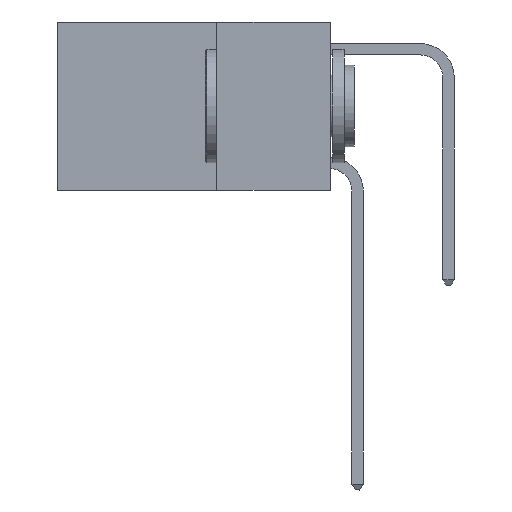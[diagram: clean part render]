
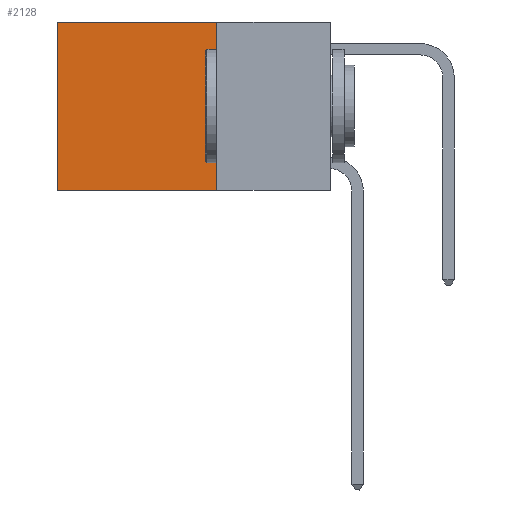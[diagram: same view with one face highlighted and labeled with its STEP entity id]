
A CAD part, left-side view. The second image highlights one B-rep face of the part: STEP entity #2128.
In plain terms, the highlighted planar face has unit normal (-1, 0, 0).
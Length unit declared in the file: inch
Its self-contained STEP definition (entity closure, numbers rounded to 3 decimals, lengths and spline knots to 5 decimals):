
#914 = EDGE_CURVE ( 'NONE', #6549, #8382, #4447, .T. ) ;
#953 = EDGE_CURVE ( 'NONE', #8583, #6549, #8649, .T. ) ;
#1019 = DIRECTION ( 'NONE',  ( 0., 0., -1. ) ) ;
#1192 = VECTOR ( 'NONE', #6654, 39.37008 ) ;
#1880 = CARTESIAN_POINT ( 'NONE',  ( 0.2625, 0.6, -0.37 ) ) ;
#2093 = VERTEX_POINT ( 'NONE', #6839 ) ;
#2128 = ADVANCED_FACE ( 'NONE', ( #10225 ), #11043, .F. ) ;
#2142 = VECTOR ( 'NONE', #7687, 39.37008 ) ;
#2522 = CARTESIAN_POINT ( 'NONE',  ( 0.2625, 0.25, 0. ) ) ;
#2741 = ORIENTED_EDGE ( 'NONE', *, *, #4528, .F. ) ;
#3237 = ORIENTED_EDGE ( 'NONE', *, *, #914, .T. ) ;
#3643 = DIRECTION ( 'NONE',  ( 1., 0., 0. ) ) ;
#3672 = ORIENTED_EDGE ( 'NONE', *, *, #5065, .F. ) ;
#3763 = LINE ( 'NONE', #7495, #1192 ) ;
#3946 = VECTOR ( 'NONE', #7718, 39.37008 ) ;
#4447 = LINE ( 'NONE', #9572, #7207 ) ;
#4528 = EDGE_CURVE ( 'NONE', #8583, #2093, #9013, .T. ) ;
#5065 = EDGE_CURVE ( 'NONE', #2093, #8382, #3763, .T. ) ;
#5420 = AXIS2_PLACEMENT_3D ( 'NONE', #8037, #3643, #1019 ) ;
#5623 = CARTESIAN_POINT ( 'NONE',  ( 0.2625, 0.25, 0. ) ) ;
#6549 = VERTEX_POINT ( 'NONE', #6883 ) ;
#6654 = DIRECTION ( 'NONE',  ( 0., 1., 0. ) ) ;
#6839 = CARTESIAN_POINT ( 'NONE',  ( 0.2625, 0.25, -0.37 ) ) ;
#6883 = CARTESIAN_POINT ( 'NONE',  ( 0.2625, 0.6, 0. ) ) ;
#7207 = VECTOR ( 'NONE', #10115, 39.37008 ) ;
#7495 = CARTESIAN_POINT ( 'NONE',  ( 0.2625, 0.25, -0.37 ) ) ;
#7581 = CARTESIAN_POINT ( 'NONE',  ( 0.2625, 0.25, 0. ) ) ;
#7687 = DIRECTION ( 'NONE',  ( 0., 0., -1. ) ) ;
#7718 = DIRECTION ( 'NONE',  ( 0., 1., 0. ) ) ;
#7970 = ORIENTED_EDGE ( 'NONE', *, *, #953, .T. ) ;
#8037 = CARTESIAN_POINT ( 'NONE',  ( 0.2625, 0.25, 0. ) ) ;
#8382 = VERTEX_POINT ( 'NONE', #1880 ) ;
#8583 = VERTEX_POINT ( 'NONE', #5623 ) ;
#8649 = LINE ( 'NONE', #7581, #3946 ) ;
#9013 = LINE ( 'NONE', #2522, #2142 ) ;
#9572 = CARTESIAN_POINT ( 'NONE',  ( 0.2625, 0.6, 0. ) ) ;
#10115 = DIRECTION ( 'NONE',  ( 0., 0., -1. ) ) ;
#10225 = FACE_OUTER_BOUND ( 'NONE', #10731, .T. ) ;
#10731 = EDGE_LOOP ( 'NONE', ( #3237, #3672, #2741, #7970 ) ) ;
#11043 = PLANE ( 'NONE',  #5420 ) ;
